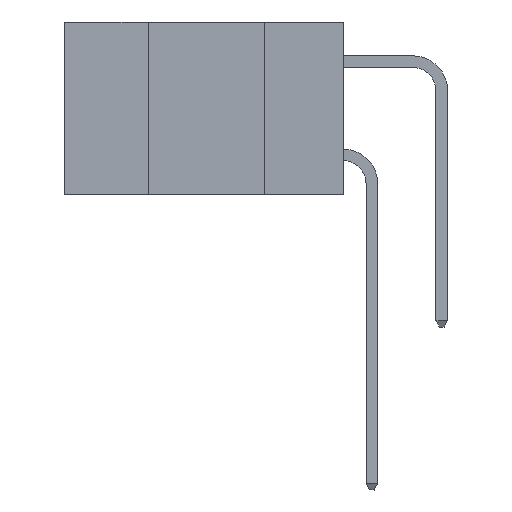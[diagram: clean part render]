
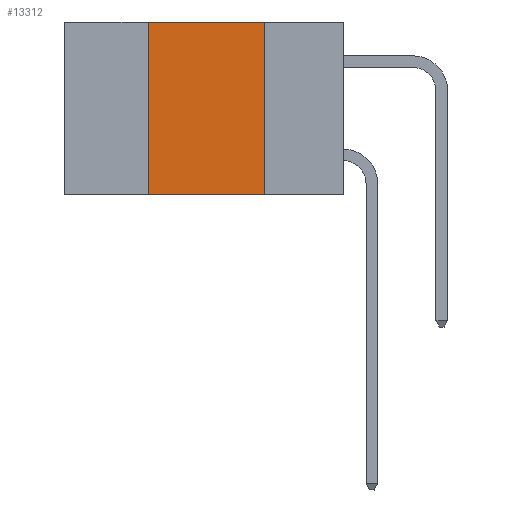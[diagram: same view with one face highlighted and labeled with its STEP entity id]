
A CAD part, left-side view. The second image highlights one B-rep face of the part: STEP entity #13312.
In plain terms, the highlighted planar face has unit normal (-1, 0, 0).
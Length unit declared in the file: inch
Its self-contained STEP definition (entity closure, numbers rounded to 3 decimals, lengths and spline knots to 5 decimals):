
#119 = EDGE_CURVE ( 'NONE', #10844, #9742, #372, .T. ) ;
#372 = LINE ( 'NONE', #6434, #7491 ) ;
#1436 = VERTEX_POINT ( 'NONE', #3774 ) ;
#1814 = EDGE_CURVE ( 'NONE', #10844, #4780, #4724, .T. ) ;
#2010 = ORIENTED_EDGE ( 'NONE', *, *, #1814, .F. ) ;
#2164 = EDGE_CURVE ( 'NONE', #1436, #9742, #4853, .T. ) ;
#2289 = VECTOR ( 'NONE', #5002, 39.37008 ) ;
#3362 = EDGE_LOOP ( 'NONE', ( #3555, #7269, #2010, #8665 ) ) ;
#3437 = CARTESIAN_POINT ( 'NONE',  ( 0., 0.17, -0.37 ) ) ;
#3555 = ORIENTED_EDGE ( 'NONE', *, *, #2164, .F. ) ;
#3774 = CARTESIAN_POINT ( 'NONE',  ( 0., 0.17, 0. ) ) ;
#4111 = LINE ( 'NONE', #15200, #13360 ) ;
#4458 = CARTESIAN_POINT ( 'NONE',  ( 0., 0.6, 0. ) ) ;
#4536 = AXIS2_PLACEMENT_3D ( 'NONE', #4458, #9335, #13917 ) ;
#4558 = DIRECTION ( 'NONE',  ( 0., -1., 0. ) ) ;
#4724 = LINE ( 'NONE', #12005, #14268 ) ;
#4780 = VERTEX_POINT ( 'NONE', #13038 ) ;
#4853 = LINE ( 'NONE', #3437, #2289 ) ;
#5002 = DIRECTION ( 'NONE',  ( 0., 0., -1. ) ) ;
#5309 = DIRECTION ( 'NONE',  ( 0., -1., 0. ) ) ;
#6434 = CARTESIAN_POINT ( 'NONE',  ( 0., 0.6, -0.37 ) ) ;
#6960 = EDGE_CURVE ( 'NONE', #4780, #1436, #4111, .T. ) ;
#7269 = ORIENTED_EDGE ( 'NONE', *, *, #6960, .F. ) ;
#7491 = VECTOR ( 'NONE', #5309, 39.37008 ) ;
#7687 = FACE_OUTER_BOUND ( 'NONE', #3362, .T. ) ;
#8665 = ORIENTED_EDGE ( 'NONE', *, *, #119, .T. ) ;
#9335 = DIRECTION ( 'NONE',  ( 1., 0., 0. ) ) ;
#9742 = VERTEX_POINT ( 'NONE', #12491 ) ;
#9839 = DIRECTION ( 'NONE',  ( 0., 0., 1. ) ) ;
#10844 = VERTEX_POINT ( 'NONE', #15553 ) ;
#11447 = PLANE ( 'NONE',  #4536 ) ;
#12005 = CARTESIAN_POINT ( 'NONE',  ( 0., 0.42, -0.37 ) ) ;
#12491 = CARTESIAN_POINT ( 'NONE',  ( 0., 0.17, -0.37 ) ) ;
#13038 = CARTESIAN_POINT ( 'NONE',  ( 0., 0.42, 0. ) ) ;
#13312 = ADVANCED_FACE ( 'NONE', ( #7687 ), #11447, .F. ) ;
#13360 = VECTOR ( 'NONE', #4558, 39.37008 ) ;
#13917 = DIRECTION ( 'NONE',  ( 0., 0., -1. ) ) ;
#14268 = VECTOR ( 'NONE', #9839, 39.37008 ) ;
#15200 = CARTESIAN_POINT ( 'NONE',  ( 0., 0.6, 0. ) ) ;
#15553 = CARTESIAN_POINT ( 'NONE',  ( 0., 0.42, -0.37 ) ) ;
